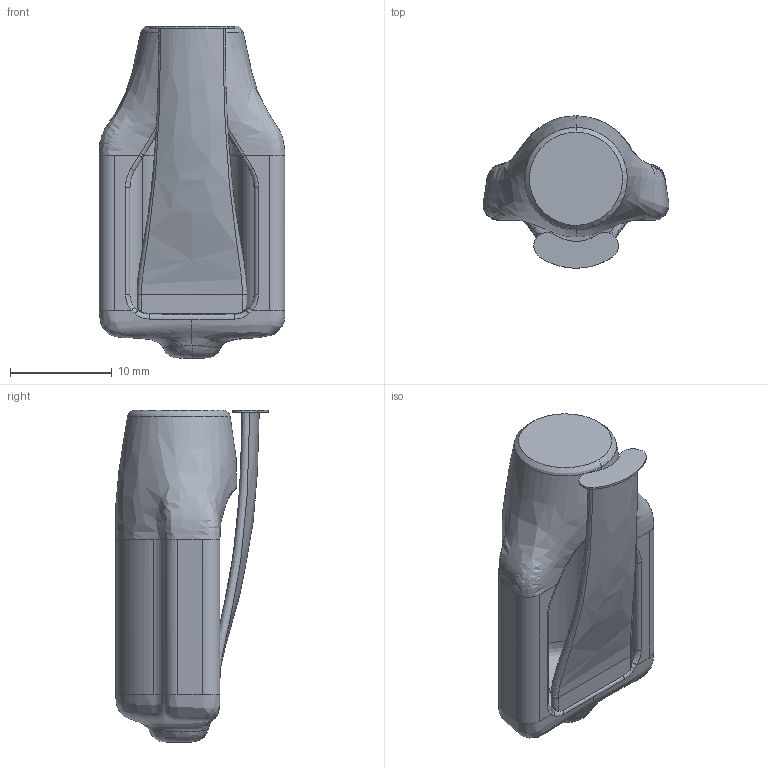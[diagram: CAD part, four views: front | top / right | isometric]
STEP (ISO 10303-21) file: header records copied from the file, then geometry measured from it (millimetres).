
FILE_DESCRIPTION (( 'STEP AP203' ), '1' );
FILE_NAME ('2.2 Hose Clamp Cover WITH SUPPORT.STEP', '2022-10-28T16:28:09', ( '' ), ( '' ), 'SwSTEP 2.0', 'SolidWorks 2021', '' );
FILE_SCHEMA (( 'CONFIG_CONTROL_DESIGN' ));
Products named in the file (1): 2.2 Hose Clamp Cover WITH SUPPORT
Bounding box: 18.25 x 14.99 x 32.61 mm (x, y, z)
Volume: 1280.4 mm3; surface area: 2962.2 mm2
Topology: 2 solids, 2 shells, 85 faces, 220 edges, 140 vertices
Faces by surface type: bspline 37, cylinder 24, plane 16, torus 8
Entity records: 52471 total; most frequent: CARTESIAN_POINT 50670, ORIENTED_EDGE 440, DIRECTION 232, EDGE_CURVE 220, VERTEX_POINT 140, B_SPLINE_CURVE_WITH_KNOTS 119, AXIS2_PLACEMENT_3D 89, EDGE_LOOP 86
